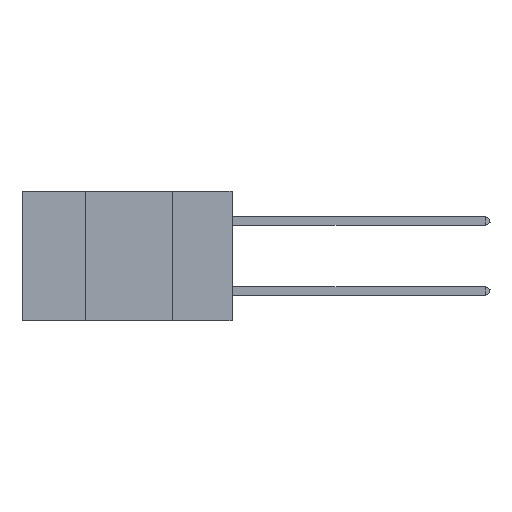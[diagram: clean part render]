
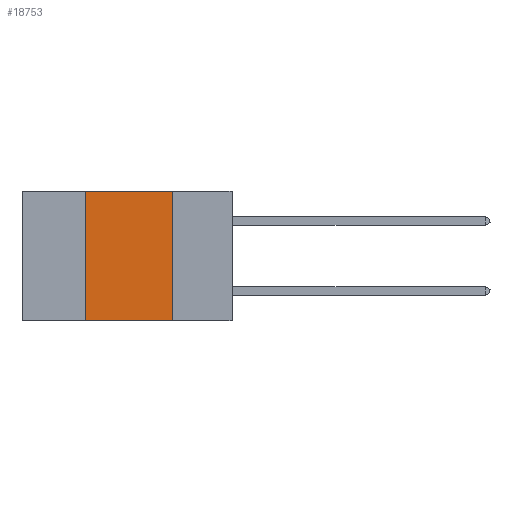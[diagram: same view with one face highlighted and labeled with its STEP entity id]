
A CAD part, left-side view. The second image highlights one B-rep face of the part: STEP entity #18753.
In plain terms, the highlighted planar face has unit normal (-1, 0, 0).
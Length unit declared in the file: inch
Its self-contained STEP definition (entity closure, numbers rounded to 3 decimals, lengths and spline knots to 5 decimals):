
#721 = EDGE_CURVE ( 'NONE', #12182, #6022, #16563, .T. ) ;
#1991 = CARTESIAN_POINT ( 'NONE',  ( 0., 0.42, 0. ) ) ;
#3079 = DIRECTION ( 'NONE',  ( 0., 0., 1. ) ) ;
#3569 = DIRECTION ( 'NONE',  ( 0., -1., 0. ) ) ;
#3662 = CARTESIAN_POINT ( 'NONE',  ( 0., 0.17, 0. ) ) ;
#4211 = LINE ( 'NONE', #10105, #20946 ) ;
#6022 = VERTEX_POINT ( 'NONE', #1991 ) ;
#6744 = ORIENTED_EDGE ( 'NONE', *, *, #9287, .F. ) ;
#7643 = FACE_OUTER_BOUND ( 'NONE', #20085, .T. ) ;
#7755 = DIRECTION ( 'NONE',  ( 0., 0., -1. ) ) ;
#9287 = EDGE_CURVE ( 'NONE', #19060, #11325, #13693, .T. ) ;
#9489 = CARTESIAN_POINT ( 'NONE',  ( 0., 0.17, 0. ) ) ;
#9535 = EDGE_CURVE ( 'NONE', #12182, #11325, #4211, .T. ) ;
#9592 = CARTESIAN_POINT ( 'NONE',  ( 0., 0.6, 0. ) ) ;
#10105 = CARTESIAN_POINT ( 'NONE',  ( 0., 0.6, -0.37 ) ) ;
#11238 = DIRECTION ( 'NONE',  ( 0., 0., -1. ) ) ;
#11325 = VERTEX_POINT ( 'NONE', #19590 ) ;
#11350 = ORIENTED_EDGE ( 'NONE', *, *, #9535, .T. ) ;
#11389 = AXIS2_PLACEMENT_3D ( 'NONE', #9592, #20855, #11238 ) ;
#12142 = CARTESIAN_POINT ( 'NONE',  ( 0., 0.42, -0.37 ) ) ;
#12182 = VERTEX_POINT ( 'NONE', #12142 ) ;
#12286 = VECTOR ( 'NONE', #3079, 39.37008 ) ;
#12437 = ORIENTED_EDGE ( 'NONE', *, *, #721, .F. ) ;
#12457 = ORIENTED_EDGE ( 'NONE', *, *, #17016, .F. ) ;
#12798 = PLANE ( 'NONE',  #11389 ) ;
#13693 = LINE ( 'NONE', #9489, #17454 ) ;
#14500 = VECTOR ( 'NONE', #20540, 39.37008 ) ;
#16563 = LINE ( 'NONE', #17988, #12286 ) ;
#17016 = EDGE_CURVE ( 'NONE', #6022, #19060, #18767, .T. ) ;
#17454 = VECTOR ( 'NONE', #7755, 39.37008 ) ;
#17988 = CARTESIAN_POINT ( 'NONE',  ( 0., 0.42, 0. ) ) ;
#18753 = ADVANCED_FACE ( 'NONE', ( #7643 ), #12798, .F. ) ;
#18767 = LINE ( 'NONE', #18933, #14500 ) ;
#18933 = CARTESIAN_POINT ( 'NONE',  ( 0., 0.6, 0. ) ) ;
#19060 = VERTEX_POINT ( 'NONE', #3662 ) ;
#19590 = CARTESIAN_POINT ( 'NONE',  ( 0., 0.17, -0.37 ) ) ;
#20085 = EDGE_LOOP ( 'NONE', ( #6744, #12457, #12437, #11350 ) ) ;
#20540 = DIRECTION ( 'NONE',  ( 0., -1., 0. ) ) ;
#20855 = DIRECTION ( 'NONE',  ( 1., 0., 0. ) ) ;
#20946 = VECTOR ( 'NONE', #3569, 39.37008 ) ;
